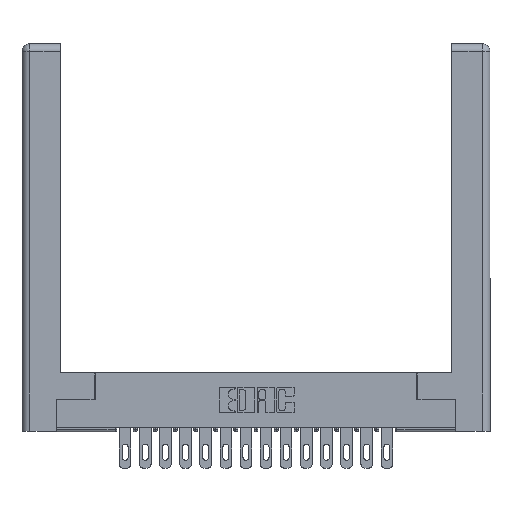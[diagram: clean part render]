
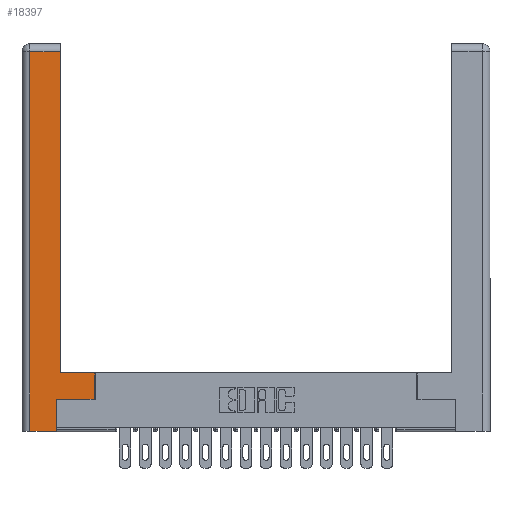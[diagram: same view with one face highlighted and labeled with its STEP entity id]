
A CAD part, top view. The second image highlights one B-rep face of the part: STEP entity #18397.
In plain terms, the highlighted planar face has unit normal (0, 0, 1).
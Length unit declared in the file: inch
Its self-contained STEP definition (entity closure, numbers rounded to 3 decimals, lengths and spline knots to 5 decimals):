
#430 = EDGE_CURVE ( 'NONE', #8822, #12530, #15850, .T. ) ;
#564 = EDGE_CURVE ( 'NONE', #12530, #16122, #8907, .T. ) ;
#1172 = CARTESIAN_POINT ( 'NONE',  ( 0.265, 0.245, 0. ) ) ;
#1899 = FACE_OUTER_BOUND ( 'NONE', #3654, .T. ) ;
#1939 = EDGE_CURVE ( 'NONE', #19151, #7145, #6060, .T. ) ;
#1999 = CARTESIAN_POINT ( 'NONE',  ( 0.565, 0.45, 0. ) ) ;
#2555 = VERTEX_POINT ( 'NONE', #6900 ) ;
#2891 = CARTESIAN_POINT ( 'NONE',  ( 0.265, 0., 0. ) ) ;
#2986 = VECTOR ( 'NONE', #12884, 39.37008 ) ;
#3017 = CARTESIAN_POINT ( 'NONE',  ( 0.565, 0.245, 0. ) ) ;
#3654 = EDGE_LOOP ( 'NONE', ( #17669, #6469, #10429, #12626, #7630, #9709, #6706, #17858 ) ) ;
#3666 = EDGE_CURVE ( 'NONE', #2555, #8822, #21154, .T. ) ;
#5129 = EDGE_CURVE ( 'NONE', #13807, #16764, #14393, .T. ) ;
#5736 = AXIS2_PLACEMENT_3D ( 'NONE', #20127, #18298, #6828 ) ;
#5815 = CARTESIAN_POINT ( 'NONE',  ( 0.295, 3., 0. ) ) ;
#5914 = CARTESIAN_POINT ( 'NONE',  ( 0.265, 0., 0. ) ) ;
#6060 = LINE ( 'NONE', #11716, #10148 ) ;
#6146 = CARTESIAN_POINT ( 'NONE',  ( 0.295, 2.94, 0. ) ) ;
#6168 = VECTOR ( 'NONE', #14019, 39.37008 ) ;
#6469 = ORIENTED_EDGE ( 'NONE', *, *, #11792, .T. ) ;
#6684 = CARTESIAN_POINT ( 'NONE',  ( 0.0615, 0., 0. ) ) ;
#6706 = ORIENTED_EDGE ( 'NONE', *, *, #3666, .T. ) ;
#6828 = DIRECTION ( 'NONE',  ( -1., 0., 0. ) ) ;
#6900 = CARTESIAN_POINT ( 'NONE',  ( 0.565, 0.245, 0. ) ) ;
#7082 = DIRECTION ( 'NONE',  ( 0., -1., 0. ) ) ;
#7145 = VERTEX_POINT ( 'NONE', #6684 ) ;
#7321 = CARTESIAN_POINT ( 'NONE',  ( 0.295, 0.45, 0. ) ) ;
#7372 = VECTOR ( 'NONE', #9244, 39.37008 ) ;
#7630 = ORIENTED_EDGE ( 'NONE', *, *, #5129, .T. ) ;
#8146 = VECTOR ( 'NONE', #18560, 39.37008 ) ;
#8519 = VECTOR ( 'NONE', #16946, 39.37008 ) ;
#8622 = LINE ( 'NONE', #3017, #9923 ) ;
#8822 = VERTEX_POINT ( 'NONE', #1999 ) ;
#8907 = LINE ( 'NONE', #5815, #7372 ) ;
#9244 = DIRECTION ( 'NONE',  ( 0., 1., 0. ) ) ;
#9369 = DIRECTION ( 'NONE',  ( 0., 1., 0. ) ) ;
#9497 = LINE ( 'NONE', #5914, #6168 ) ;
#9709 = ORIENTED_EDGE ( 'NONE', *, *, #11224, .T. ) ;
#9923 = VECTOR ( 'NONE', #12744, 39.37008 ) ;
#10148 = VECTOR ( 'NONE', #7082, 39.37008 ) ;
#10195 = PLANE ( 'NONE',  #5736 ) ;
#10429 = ORIENTED_EDGE ( 'NONE', *, *, #1939, .T. ) ;
#11224 = EDGE_CURVE ( 'NONE', #16764, #2555, #8622, .T. ) ;
#11716 = CARTESIAN_POINT ( 'NONE',  ( 0.0615, 0., 0. ) ) ;
#11792 = EDGE_CURVE ( 'NONE', #16122, #19151, #12426, .T. ) ;
#12426 = LINE ( 'NONE', #21105, #2986 ) ;
#12530 = VERTEX_POINT ( 'NONE', #17082 ) ;
#12626 = ORIENTED_EDGE ( 'NONE', *, *, #20784, .T. ) ;
#12744 = DIRECTION ( 'NONE',  ( 1., 0., 0. ) ) ;
#12884 = DIRECTION ( 'NONE',  ( -1., 0., 0. ) ) ;
#13790 = CARTESIAN_POINT ( 'NONE',  ( 0.565, 0.45, 0. ) ) ;
#13807 = VERTEX_POINT ( 'NONE', #2891 ) ;
#14019 = DIRECTION ( 'NONE',  ( 1., 0., 0. ) ) ;
#14393 = LINE ( 'NONE', #14469, #20576 ) ;
#14469 = CARTESIAN_POINT ( 'NONE',  ( 0.265, 0.245, 0. ) ) ;
#15850 = LINE ( 'NONE', #7321, #8146 ) ;
#16122 = VERTEX_POINT ( 'NONE', #6146 ) ;
#16764 = VERTEX_POINT ( 'NONE', #1172 ) ;
#16946 = DIRECTION ( 'NONE',  ( 0., 1., 0. ) ) ;
#17035 = CARTESIAN_POINT ( 'NONE',  ( 0.0615, 2.94, 0. ) ) ;
#17082 = CARTESIAN_POINT ( 'NONE',  ( 0.295, 0.45, 0. ) ) ;
#17669 = ORIENTED_EDGE ( 'NONE', *, *, #564, .T. ) ;
#17858 = ORIENTED_EDGE ( 'NONE', *, *, #430, .T. ) ;
#18298 = DIRECTION ( 'NONE',  ( 0., 0., -1. ) ) ;
#18397 = ADVANCED_FACE ( 'NONE', ( #1899 ), #10195, .F. ) ;
#18560 = DIRECTION ( 'NONE',  ( -1., 0., 0. ) ) ;
#19151 = VERTEX_POINT ( 'NONE', #17035 ) ;
#20127 = CARTESIAN_POINT ( 'NONE',  ( 0., 0., 0. ) ) ;
#20576 = VECTOR ( 'NONE', #9369, 39.37008 ) ;
#20784 = EDGE_CURVE ( 'NONE', #7145, #13807, #9497, .T. ) ;
#21105 = CARTESIAN_POINT ( 'NONE',  ( 0.0615, 2.94, 0. ) ) ;
#21154 = LINE ( 'NONE', #13790, #8519 ) ;
